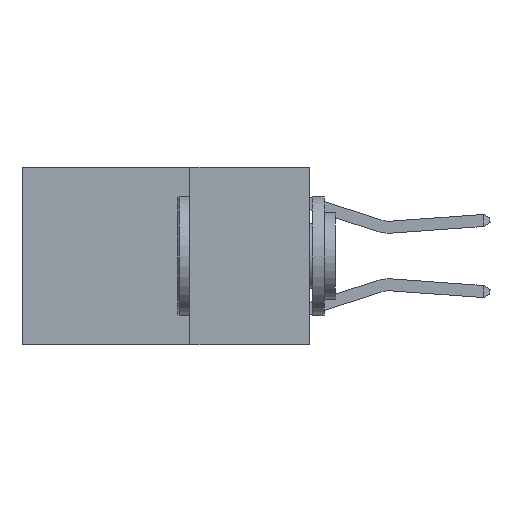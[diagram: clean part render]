
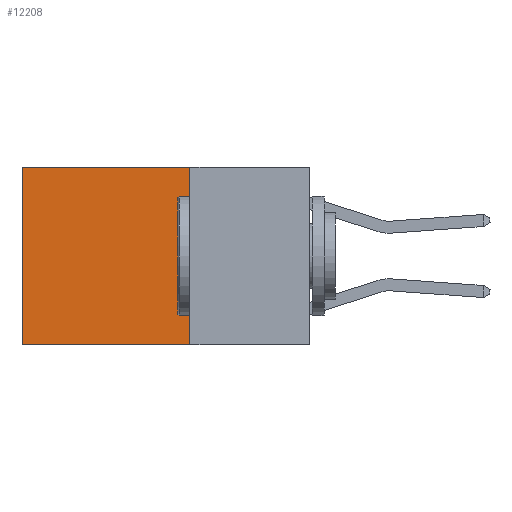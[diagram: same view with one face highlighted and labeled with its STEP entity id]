
A CAD part, left-side view. The second image highlights one B-rep face of the part: STEP entity #12208.
In plain terms, the highlighted planar face has unit normal (-1, 0, 0).
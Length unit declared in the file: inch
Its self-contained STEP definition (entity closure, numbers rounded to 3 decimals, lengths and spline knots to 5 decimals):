
#340 = EDGE_CURVE ( 'NONE', #9225, #12495, #17909, .T. ) ;
#1367 = EDGE_LOOP ( 'NONE', ( #16463, #14233, #24014, #1744 ) ) ;
#1686 = CARTESIAN_POINT ( 'NONE',  ( 0.2625, 0.25, 0. ) ) ;
#1744 = ORIENTED_EDGE ( 'NONE', *, *, #16556, .T. ) ;
#1906 = VERTEX_POINT ( 'NONE', #22592 ) ;
#5108 = LINE ( 'NONE', #10916, #15230 ) ;
#6587 = CARTESIAN_POINT ( 'NONE',  ( 0.2625, 0.6, 0. ) ) ;
#7037 = CARTESIAN_POINT ( 'NONE',  ( 0.2625, 0.25, 0. ) ) ;
#7125 = PLANE ( 'NONE',  #14759 ) ;
#7165 = CARTESIAN_POINT ( 'NONE',  ( 0.2625, 0.25, -0.37 ) ) ;
#9225 = VERTEX_POINT ( 'NONE', #7037 ) ;
#10916 = CARTESIAN_POINT ( 'NONE',  ( 0.2625, 0.25, 0. ) ) ;
#12208 = ADVANCED_FACE ( 'NONE', ( #18537 ), #7125, .F. ) ;
#12320 = DIRECTION ( 'NONE',  ( 0., 0., -1. ) ) ;
#12495 = VERTEX_POINT ( 'NONE', #21621 ) ;
#12600 = VERTEX_POINT ( 'NONE', #23849 ) ;
#14183 = DIRECTION ( 'NONE',  ( 0., 0., -1. ) ) ;
#14233 = ORIENTED_EDGE ( 'NONE', *, *, #15770, .F. ) ;
#14759 = AXIS2_PLACEMENT_3D ( 'NONE', #1686, #18899, #17050 ) ;
#15208 = EDGE_CURVE ( 'NONE', #1906, #12600, #16050, .T. ) ;
#15230 = VECTOR ( 'NONE', #20119, 39.37008 ) ;
#15770 = EDGE_CURVE ( 'NONE', #12495, #12600, #24161, .T. ) ;
#16050 = LINE ( 'NONE', #6587, #23495 ) ;
#16173 = CARTESIAN_POINT ( 'NONE',  ( 0.2625, 0.25, 0. ) ) ;
#16463 = ORIENTED_EDGE ( 'NONE', *, *, #15208, .T. ) ;
#16556 = EDGE_CURVE ( 'NONE', #9225, #1906, #5108, .T. ) ;
#17050 = DIRECTION ( 'NONE',  ( 0., 0., -1. ) ) ;
#17909 = LINE ( 'NONE', #16173, #19835 ) ;
#18105 = DIRECTION ( 'NONE',  ( 0., 1., 0. ) ) ;
#18537 = FACE_OUTER_BOUND ( 'NONE', #1367, .T. ) ;
#18899 = DIRECTION ( 'NONE',  ( 1., 0., 0. ) ) ;
#19835 = VECTOR ( 'NONE', #12320, 39.37008 ) ;
#20119 = DIRECTION ( 'NONE',  ( 0., 1., 0. ) ) ;
#21133 = VECTOR ( 'NONE', #18105, 39.37008 ) ;
#21621 = CARTESIAN_POINT ( 'NONE',  ( 0.2625, 0.25, -0.37 ) ) ;
#22592 = CARTESIAN_POINT ( 'NONE',  ( 0.2625, 0.6, 0. ) ) ;
#23495 = VECTOR ( 'NONE', #14183, 39.37008 ) ;
#23849 = CARTESIAN_POINT ( 'NONE',  ( 0.2625, 0.6, -0.37 ) ) ;
#24014 = ORIENTED_EDGE ( 'NONE', *, *, #340, .F. ) ;
#24161 = LINE ( 'NONE', #7165, #21133 ) ;
